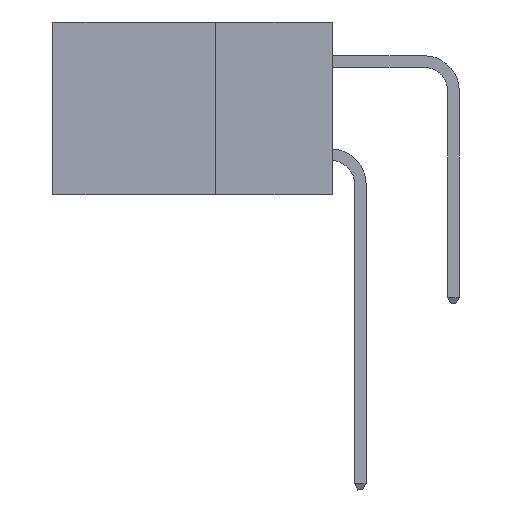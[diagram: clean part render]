
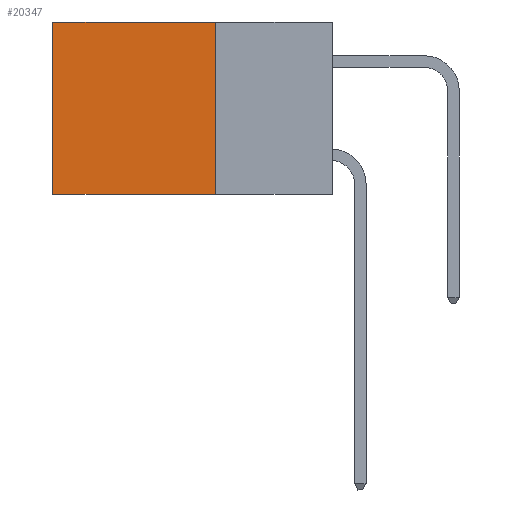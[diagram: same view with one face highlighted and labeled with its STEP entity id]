
A CAD part, left-side view. The second image highlights one B-rep face of the part: STEP entity #20347.
In plain terms, the highlighted planar face has unit normal (-1, 0, 0).
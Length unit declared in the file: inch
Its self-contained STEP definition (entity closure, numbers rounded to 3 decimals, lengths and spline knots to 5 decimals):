
#135 = AXIS2_PLACEMENT_3D ( 'NONE', #5165, #7174, #20802 ) ;
#1071 = CARTESIAN_POINT ( 'NONE',  ( 0.2615, 0.6, -0.37 ) ) ;
#1462 = VECTOR ( 'NONE', #19759, 39.37008 ) ;
#1991 = VECTOR ( 'NONE', #5862, 39.37008 ) ;
#2071 = EDGE_CURVE ( 'NONE', #21398, #5412, #12394, .T. ) ;
#2136 = ORIENTED_EDGE ( 'NONE', *, *, #2071, .T. ) ;
#3224 = LINE ( 'NONE', #5114, #17622 ) ;
#4284 = CARTESIAN_POINT ( 'NONE',  ( 0.2615, 0.6, 0. ) ) ;
#4448 = CARTESIAN_POINT ( 'NONE',  ( 0.2615, 0.25, -0.37 ) ) ;
#4937 = FACE_OUTER_BOUND ( 'NONE', #15511, .T. ) ;
#5114 = CARTESIAN_POINT ( 'NONE',  ( 0.2615, 0.25, 0. ) ) ;
#5165 = CARTESIAN_POINT ( 'NONE',  ( 0.2615, 0.25, -0.37 ) ) ;
#5257 = VECTOR ( 'NONE', #6429, 39.37008 ) ;
#5299 = CARTESIAN_POINT ( 'NONE',  ( 0.2615, 0.6, -0.37 ) ) ;
#5412 = VERTEX_POINT ( 'NONE', #1071 ) ;
#5862 = DIRECTION ( 'NONE',  ( 0., 0., -1. ) ) ;
#6092 = CARTESIAN_POINT ( 'NONE',  ( 0.2615, 0.25, -0.37 ) ) ;
#6429 = DIRECTION ( 'NONE',  ( 0., 0., -1. ) ) ;
#6670 = LINE ( 'NONE', #6092, #1462 ) ;
#7119 = DIRECTION ( 'NONE',  ( 0., 1., 0. ) ) ;
#7174 = DIRECTION ( 'NONE',  ( 1., 0., 0. ) ) ;
#8706 = CARTESIAN_POINT ( 'NONE',  ( 0.2615, 0.25, -0.37 ) ) ;
#9006 = CARTESIAN_POINT ( 'NONE',  ( 0.2615, 0.25, 0. ) ) ;
#12394 = LINE ( 'NONE', #5299, #1991 ) ;
#12854 = VERTEX_POINT ( 'NONE', #8706 ) ;
#13416 = VERTEX_POINT ( 'NONE', #9006 ) ;
#14342 = ORIENTED_EDGE ( 'NONE', *, *, #24060, .T. ) ;
#15366 = ORIENTED_EDGE ( 'NONE', *, *, #19411, .F. ) ;
#15511 = EDGE_LOOP ( 'NONE', ( #2136, #19748, #15366, #14342 ) ) ;
#16426 = EDGE_CURVE ( 'NONE', #12854, #5412, #6670, .T. ) ;
#17622 = VECTOR ( 'NONE', #7119, 39.37008 ) ;
#18874 = PLANE ( 'NONE',  #135 ) ;
#19411 = EDGE_CURVE ( 'NONE', #13416, #12854, #20838, .T. ) ;
#19748 = ORIENTED_EDGE ( 'NONE', *, *, #16426, .F. ) ;
#19759 = DIRECTION ( 'NONE',  ( 0., 1., 0. ) ) ;
#20347 = ADVANCED_FACE ( 'NONE', ( #4937 ), #18874, .F. ) ;
#20802 = DIRECTION ( 'NONE',  ( 0., 0., -1. ) ) ;
#20838 = LINE ( 'NONE', #4448, #5257 ) ;
#21398 = VERTEX_POINT ( 'NONE', #4284 ) ;
#24060 = EDGE_CURVE ( 'NONE', #13416, #21398, #3224, .T. ) ;
